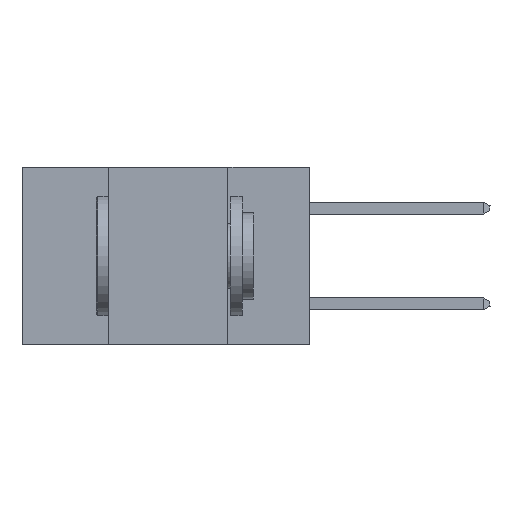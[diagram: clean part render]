
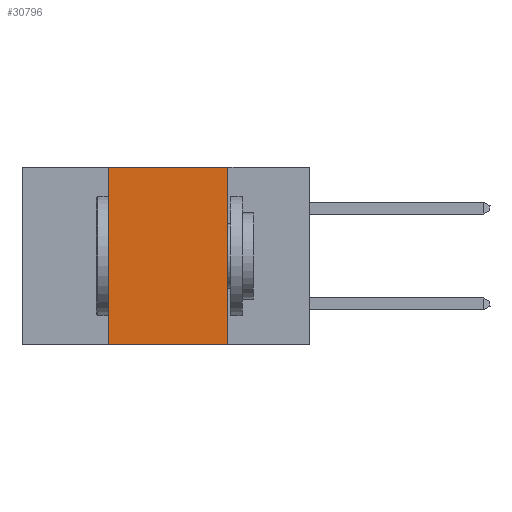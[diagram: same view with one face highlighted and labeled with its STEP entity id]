
A CAD part, left-side view. The second image highlights one B-rep face of the part: STEP entity #30796.
In plain terms, the highlighted planar face has unit normal (-1, 0, 0).
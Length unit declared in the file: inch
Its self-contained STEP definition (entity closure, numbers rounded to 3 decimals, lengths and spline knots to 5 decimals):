
#477 = CARTESIAN_POINT ( 'NONE',  ( 0., 0.6, 0. ) ) ;
#484 = LINE ( 'NONE', #477, #34612 ) ;
#713 = FACE_OUTER_BOUND ( 'NONE', #21973, .T. ) ;
#3232 = VERTEX_POINT ( 'NONE', #36412 ) ;
#3544 = CARTESIAN_POINT ( 'NONE',  ( 0., 0.17, 0. ) ) ;
#5298 = AXIS2_PLACEMENT_3D ( 'NONE', #38640, #20003, #38356 ) ;
#7634 = CARTESIAN_POINT ( 'NONE',  ( 0., 0.42, 0. ) ) ;
#9411 = VERTEX_POINT ( 'NONE', #7634 ) ;
#10718 = EDGE_CURVE ( 'NONE', #3232, #11274, #30265, .T. ) ;
#11274 = VERTEX_POINT ( 'NONE', #32151 ) ;
#13564 = PLANE ( 'NONE',  #5298 ) ;
#13910 = CARTESIAN_POINT ( 'NONE',  ( 0., 0.42, 0. ) ) ;
#14218 = EDGE_CURVE ( 'NONE', #32306, #11274, #33973, .T. ) ;
#16733 = VECTOR ( 'NONE', #29628, 39.37008 ) ;
#16966 = EDGE_CURVE ( 'NONE', #3232, #9411, #34289, .T. ) ;
#19247 = CARTESIAN_POINT ( 'NONE',  ( 0., 0.17, 0. ) ) ;
#20003 = DIRECTION ( 'NONE',  ( 1., 0., 0. ) ) ;
#20350 = CARTESIAN_POINT ( 'NONE',  ( 0., 0.6, -0.37 ) ) ;
#21973 = EDGE_LOOP ( 'NONE', ( #24422, #28934, #36406, #28378 ) ) ;
#22787 = VECTOR ( 'NONE', #31803, 39.37008 ) ;
#24422 = ORIENTED_EDGE ( 'NONE', *, *, #14218, .F. ) ;
#26899 = VECTOR ( 'NONE', #29351, 39.37008 ) ;
#28378 = ORIENTED_EDGE ( 'NONE', *, *, #10718, .T. ) ;
#28934 = ORIENTED_EDGE ( 'NONE', *, *, #33729, .F. ) ;
#29351 = DIRECTION ( 'NONE',  ( 0., -1., 0. ) ) ;
#29628 = DIRECTION ( 'NONE',  ( 0., 0., 1. ) ) ;
#30265 = LINE ( 'NONE', #20350, #26899 ) ;
#30796 = ADVANCED_FACE ( 'NONE', ( #713 ), #13564, .F. ) ;
#31384 = DIRECTION ( 'NONE',  ( 0., -1., 0. ) ) ;
#31803 = DIRECTION ( 'NONE',  ( 0., 0., -1. ) ) ;
#32151 = CARTESIAN_POINT ( 'NONE',  ( 0., 0.17, -0.37 ) ) ;
#32306 = VERTEX_POINT ( 'NONE', #3544 ) ;
#33729 = EDGE_CURVE ( 'NONE', #9411, #32306, #484, .T. ) ;
#33973 = LINE ( 'NONE', #19247, #22787 ) ;
#34289 = LINE ( 'NONE', #13910, #16733 ) ;
#34612 = VECTOR ( 'NONE', #31384, 39.37008 ) ;
#36406 = ORIENTED_EDGE ( 'NONE', *, *, #16966, .F. ) ;
#36412 = CARTESIAN_POINT ( 'NONE',  ( 0., 0.42, -0.37 ) ) ;
#38356 = DIRECTION ( 'NONE',  ( 0., 0., -1. ) ) ;
#38640 = CARTESIAN_POINT ( 'NONE',  ( 0., 0.6, 0. ) ) ;
